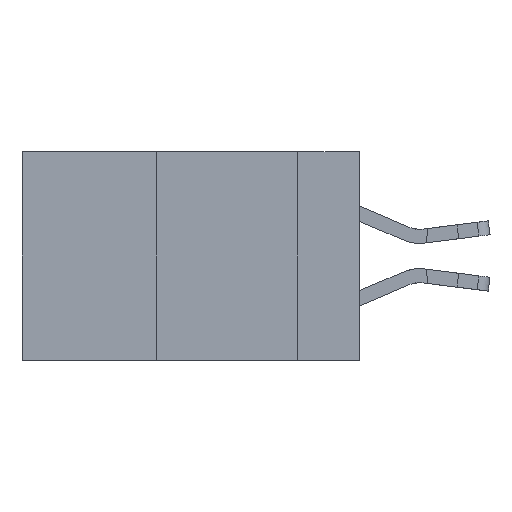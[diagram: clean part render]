
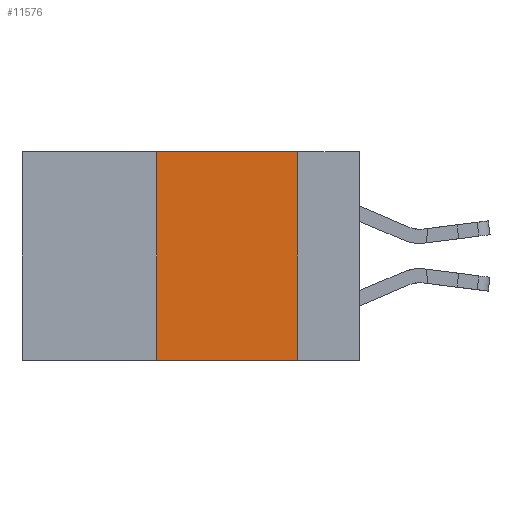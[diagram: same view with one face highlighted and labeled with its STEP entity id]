
A CAD part, left-side view. The second image highlights one B-rep face of the part: STEP entity #11576.
In plain terms, the highlighted planar face has unit normal (-1, 0, 0).
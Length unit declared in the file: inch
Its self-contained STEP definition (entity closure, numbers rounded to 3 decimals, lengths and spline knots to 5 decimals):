
#348 = DIRECTION ( 'NONE',  ( 0., -1., 0. ) ) ;
#423 = DIRECTION ( 'NONE',  ( 1., 0., 0. ) ) ;
#1632 = DIRECTION ( 'NONE',  ( 0., -1., 0. ) ) ;
#1670 = EDGE_CURVE ( 'NONE', #6324, #16168, #1714, .T. ) ;
#1714 = LINE ( 'NONE', #1778, #14868 ) ;
#1778 = CARTESIAN_POINT ( 'NONE',  ( 0., 0.6, -0.37 ) ) ;
#3446 = EDGE_CURVE ( 'NONE', #6324, #12300, #11434, .T. ) ;
#3618 = DIRECTION ( 'NONE',  ( 0., 0., 1. ) ) ;
#4530 = CARTESIAN_POINT ( 'NONE',  ( 0., 0.36, 0. ) ) ;
#5134 = AXIS2_PLACEMENT_3D ( 'NONE', #8522, #423, #9839 ) ;
#5664 = ORIENTED_EDGE ( 'NONE', *, *, #1670, .T. ) ;
#6324 = VERTEX_POINT ( 'NONE', #8647 ) ;
#7997 = VECTOR ( 'NONE', #3618, 39.37008 ) ;
#8522 = CARTESIAN_POINT ( 'NONE',  ( 0., 0.6, 0. ) ) ;
#8647 = CARTESIAN_POINT ( 'NONE',  ( 0., 0.36, -0.37 ) ) ;
#9459 = FACE_OUTER_BOUND ( 'NONE', #13513, .T. ) ;
#9694 = VERTEX_POINT ( 'NONE', #12745 ) ;
#9761 = EDGE_CURVE ( 'NONE', #9694, #16168, #14098, .T. ) ;
#9776 = PLANE ( 'NONE',  #5134 ) ;
#9839 = DIRECTION ( 'NONE',  ( 0., 0., -1. ) ) ;
#10666 = VECTOR ( 'NONE', #1632, 39.37008 ) ;
#11434 = LINE ( 'NONE', #14090, #7997 ) ;
#11447 = ORIENTED_EDGE ( 'NONE', *, *, #3446, .F. ) ;
#11500 = EDGE_CURVE ( 'NONE', #12300, #9694, #14041, .T. ) ;
#11576 = ADVANCED_FACE ( 'NONE', ( #9459 ), #9776, .F. ) ;
#11639 = ORIENTED_EDGE ( 'NONE', *, *, #9761, .F. ) ;
#12300 = VERTEX_POINT ( 'NONE', #4530 ) ;
#12745 = CARTESIAN_POINT ( 'NONE',  ( 0., 0.11, 0. ) ) ;
#12857 = CARTESIAN_POINT ( 'NONE',  ( 0., 0.11, 0. ) ) ;
#13220 = CARTESIAN_POINT ( 'NONE',  ( 0., 0.11, -0.37 ) ) ;
#13450 = CARTESIAN_POINT ( 'NONE',  ( 0., 0.6, 0. ) ) ;
#13513 = EDGE_LOOP ( 'NONE', ( #11639, #14038, #11447, #5664 ) ) ;
#13684 = VECTOR ( 'NONE', #14140, 39.37008 ) ;
#14038 = ORIENTED_EDGE ( 'NONE', *, *, #11500, .F. ) ;
#14041 = LINE ( 'NONE', #13450, #10666 ) ;
#14090 = CARTESIAN_POINT ( 'NONE',  ( 0., 0.36, 0. ) ) ;
#14098 = LINE ( 'NONE', #12857, #13684 ) ;
#14140 = DIRECTION ( 'NONE',  ( 0., 0., -1. ) ) ;
#14868 = VECTOR ( 'NONE', #348, 39.37008 ) ;
#16168 = VERTEX_POINT ( 'NONE', #13220 ) ;
